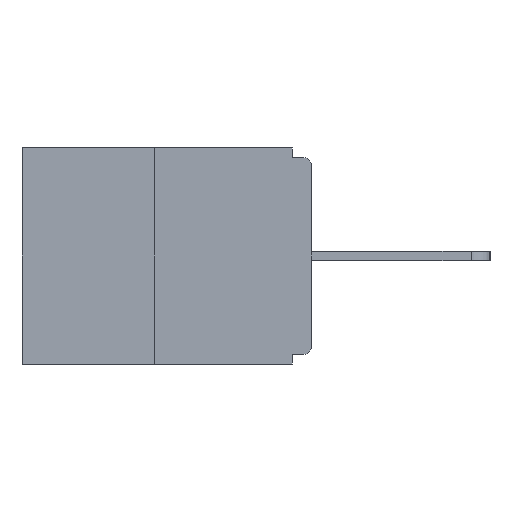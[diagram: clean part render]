
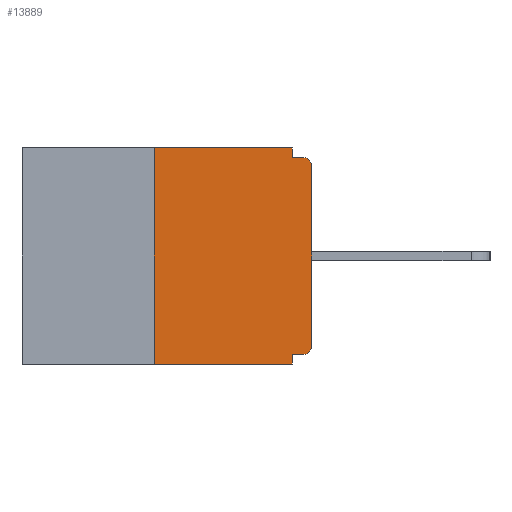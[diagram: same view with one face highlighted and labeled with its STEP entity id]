
A CAD part, left-side view. The second image highlights one B-rep face of the part: STEP entity #13889.
In plain terms, the highlighted planar face has unit normal (-1, 0, 0).
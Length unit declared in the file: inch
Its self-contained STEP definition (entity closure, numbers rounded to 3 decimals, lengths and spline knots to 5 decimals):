
#37 = VERTEX_POINT ( 'NONE', #7096 ) ;
#163 = EDGE_LOOP ( 'NONE', ( #12864, #5835, #10147, #19253, #12360, #14193, #20233, #5192, #4966, #12798 ) ) ;
#760 = DIRECTION ( 'NONE',  ( 0., 1., 0. ) ) ;
#1201 = VERTEX_POINT ( 'NONE', #13503 ) ;
#1324 = VERTEX_POINT ( 'NONE', #15870 ) ;
#1427 = DIRECTION ( 'NONE',  ( 0., -1., 0. ) ) ;
#1576 = EDGE_CURVE ( 'NONE', #17418, #1201, #21979, .T. ) ;
#1712 = DIRECTION ( 'NONE',  ( 0., 0., -1. ) ) ;
#2048 = CARTESIAN_POINT ( 'NONE',  ( 0., 0.015, -0.313 ) ) ;
#2732 = DIRECTION ( 'NONE',  ( -1., 0., 0. ) ) ;
#3101 = CARTESIAN_POINT ( 'NONE',  ( 0., 0.46, -0.343 ) ) ;
#3111 = LINE ( 'NONE', #11577, #10711 ) ;
#3212 = EDGE_CURVE ( 'NONE', #20468, #37, #13240, .T. ) ;
#3453 = CARTESIAN_POINT ( 'NONE',  ( 0., 0.46, 0. ) ) ;
#3680 = CARTESIAN_POINT ( 'NONE',  ( 0., 0.015, -0.328 ) ) ;
#4187 = DIRECTION ( 'NONE',  ( 0., 0., -1. ) ) ;
#4275 = EDGE_CURVE ( 'NONE', #1201, #10885, #20052, .T. ) ;
#4546 = CIRCLE ( 'NONE', #18813, 0.015 ) ;
#4726 = CARTESIAN_POINT ( 'NONE',  ( 0., 0.25, -0.343 ) ) ;
#4966 = ORIENTED_EDGE ( 'NONE', *, *, #16414, .F. ) ;
#5192 = ORIENTED_EDGE ( 'NONE', *, *, #18664, .T. ) ;
#5289 = EDGE_CURVE ( 'NONE', #16576, #15022, #11097, .T. ) ;
#5413 = CARTESIAN_POINT ( 'NONE',  ( 0., 0.25, 0. ) ) ;
#5604 = AXIS2_PLACEMENT_3D ( 'NONE', #14226, #5738, #4187 ) ;
#5738 = DIRECTION ( 'NONE',  ( 1., 0., 0. ) ) ;
#5835 = ORIENTED_EDGE ( 'NONE', *, *, #12990, .F. ) ;
#6276 = VECTOR ( 'NONE', #16060, 39.37008 ) ;
#7096 = CARTESIAN_POINT ( 'NONE',  ( 0., 0.031, -0.343 ) ) ;
#7405 = PLANE ( 'NONE',  #5604 ) ;
#7746 = VECTOR ( 'NONE', #18452, 39.37008 ) ;
#8847 = VERTEX_POINT ( 'NONE', #14413 ) ;
#8851 = DIRECTION ( 'NONE',  ( -1., 0., 0. ) ) ;
#8958 = DIRECTION ( 'NONE',  ( 0., 0., -1. ) ) ;
#9079 = CARTESIAN_POINT ( 'NONE',  ( 0., 0., -0.03 ) ) ;
#9708 = CARTESIAN_POINT ( 'NONE',  ( 0., 0., -0.015 ) ) ;
#9995 = DIRECTION ( 'NONE',  ( 0., -1., 0. ) ) ;
#10147 = ORIENTED_EDGE ( 'NONE', *, *, #3212, .T. ) ;
#10711 = VECTOR ( 'NONE', #13366, 39.37008 ) ;
#10885 = VERTEX_POINT ( 'NONE', #20311 ) ;
#11097 = LINE ( 'NONE', #21607, #17884 ) ;
#11577 = CARTESIAN_POINT ( 'NONE',  ( 0., 0.031, -0.343 ) ) ;
#11723 = LINE ( 'NONE', #9708, #7746 ) ;
#12360 = ORIENTED_EDGE ( 'NONE', *, *, #14278, .F. ) ;
#12587 = LINE ( 'NONE', #14599, #17050 ) ;
#12798 = ORIENTED_EDGE ( 'NONE', *, *, #4275, .F. ) ;
#12864 = ORIENTED_EDGE ( 'NONE', *, *, #1576, .F. ) ;
#12990 = EDGE_CURVE ( 'NONE', #20468, #17418, #19307, .T. ) ;
#13240 = LINE ( 'NONE', #3101, #14983 ) ;
#13366 = DIRECTION ( 'NONE',  ( 0., 0., -1. ) ) ;
#13503 = CARTESIAN_POINT ( 'NONE',  ( 0., 0.031, 0. ) ) ;
#13770 = VECTOR ( 'NONE', #1427, 39.37008 ) ;
#13869 = EDGE_CURVE ( 'NONE', #15509, #16576, #4546, .T. ) ;
#13889 = ADVANCED_FACE ( 'NONE', ( #20937 ), #7405, .F. ) ;
#13939 = CIRCLE ( 'NONE', #14287, 0.015 ) ;
#14193 = ORIENTED_EDGE ( 'NONE', *, *, #13869, .T. ) ;
#14226 = CARTESIAN_POINT ( 'NONE',  ( 0., 0.46, 0. ) ) ;
#14270 = CARTESIAN_POINT ( 'NONE',  ( 0., 0.25, 0. ) ) ;
#14278 = EDGE_CURVE ( 'NONE', #15509, #1324, #12587, .T. ) ;
#14287 = AXIS2_PLACEMENT_3D ( 'NONE', #18143, #2732, #16242 ) ;
#14413 = CARTESIAN_POINT ( 'NONE',  ( 0., 0.015, -0.015 ) ) ;
#14599 = CARTESIAN_POINT ( 'NONE',  ( 0., 0., -0.328 ) ) ;
#14983 = VECTOR ( 'NONE', #9995, 39.37008 ) ;
#15022 = VERTEX_POINT ( 'NONE', #9079 ) ;
#15509 = VERTEX_POINT ( 'NONE', #3680 ) ;
#15608 = VECTOR ( 'NONE', #1712, 39.37008 ) ;
#15870 = CARTESIAN_POINT ( 'NONE',  ( 0., 0.031, -0.328 ) ) ;
#16060 = DIRECTION ( 'NONE',  ( 0., 0., 1. ) ) ;
#16242 = DIRECTION ( 'NONE',  ( 0., 0., -1. ) ) ;
#16414 = EDGE_CURVE ( 'NONE', #10885, #8847, #11723, .T. ) ;
#16576 = VERTEX_POINT ( 'NONE', #17544 ) ;
#17050 = VECTOR ( 'NONE', #760, 39.37008 ) ;
#17418 = VERTEX_POINT ( 'NONE', #5413 ) ;
#17544 = CARTESIAN_POINT ( 'NONE',  ( 0., 0., -0.313 ) ) ;
#17884 = VECTOR ( 'NONE', #19944, 39.37008 ) ;
#18143 = CARTESIAN_POINT ( 'NONE',  ( 0., 0.015, -0.03 ) ) ;
#18452 = DIRECTION ( 'NONE',  ( 0., -1., 0. ) ) ;
#18474 = EDGE_CURVE ( 'NONE', #1324, #37, #3111, .T. ) ;
#18664 = EDGE_CURVE ( 'NONE', #15022, #8847, #13939, .T. ) ;
#18813 = AXIS2_PLACEMENT_3D ( 'NONE', #2048, #8851, #8958 ) ;
#19253 = ORIENTED_EDGE ( 'NONE', *, *, #18474, .F. ) ;
#19307 = LINE ( 'NONE', #14270, #6276 ) ;
#19944 = DIRECTION ( 'NONE',  ( 0., 0., 1. ) ) ;
#20052 = LINE ( 'NONE', #22041, #15608 ) ;
#20233 = ORIENTED_EDGE ( 'NONE', *, *, #5289, .T. ) ;
#20311 = CARTESIAN_POINT ( 'NONE',  ( 0., 0.031, -0.015 ) ) ;
#20468 = VERTEX_POINT ( 'NONE', #4726 ) ;
#20937 = FACE_OUTER_BOUND ( 'NONE', #163, .T. ) ;
#21607 = CARTESIAN_POINT ( 'NONE',  ( 0., 0., 0. ) ) ;
#21979 = LINE ( 'NONE', #3453, #13770 ) ;
#22041 = CARTESIAN_POINT ( 'NONE',  ( 0., 0.031, 0. ) ) ;
